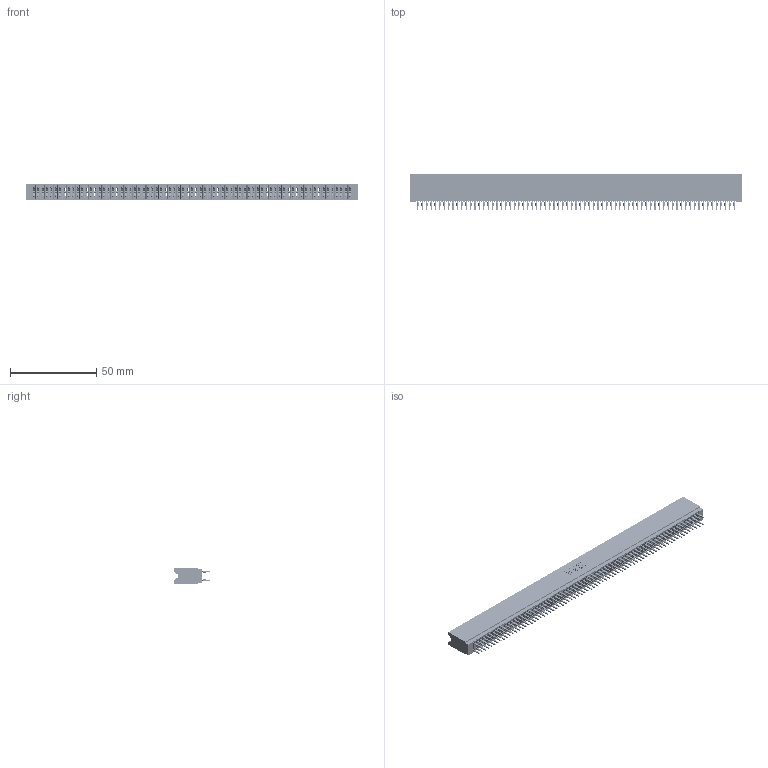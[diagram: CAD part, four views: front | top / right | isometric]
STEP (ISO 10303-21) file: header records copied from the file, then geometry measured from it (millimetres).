
FILE_DESCRIPTION (( 'STEP AP203' ), '1' );
FILE_NAME ('745-146-520-206.STEP', '2020-09-15T12:52:18', ( '' ), ( '' ), 'SwSTEP 2.0', 'SolidWorks 2020', '' );
FILE_SCHEMA (( 'CONFIG_CONTROL_DESIGN' ));
Length unit declared in the file: inch
Products named in the file (3): 745-292-001_520; 745 Part_Insulator Option - 06; 745-146-520-206
Assembly tree (147 placements, depth 2):
  745-146-520-206
    745 Part_Insulator Option - 06
    745-292-001_520  x146
Bounding box: 192.02 x 21.22 x 8.89 mm (x, y, z)
Volume: 16961.2 mm3; surface area: 34551.3 mm2
Topology: 147 solids, 147 shells, 13163 faces, 35373 edges, 22218 vertices
Faces by surface type: plane 6772, bspline 2920, cylinder 2595, torus 876
Entity records: 118691 total; most frequent: CARTESIAN_POINT 21078, ORIENTED_EDGE 20576, DIRECTION 17948, EDGE_CURVE 10288, LINE 9668, VECTOR 9668, VERTEX_POINT 6558, AXIS2_PLACEMENT_3D 4140
